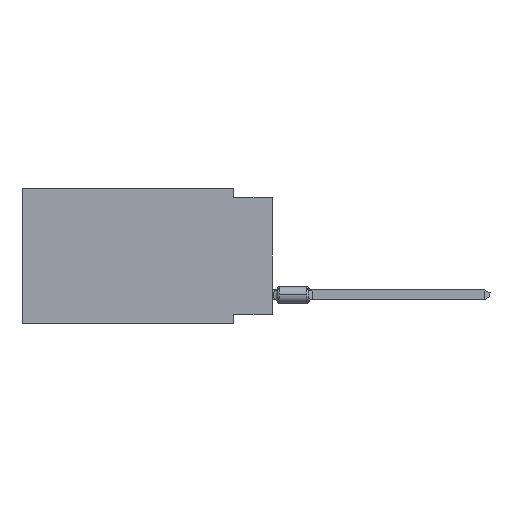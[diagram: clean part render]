
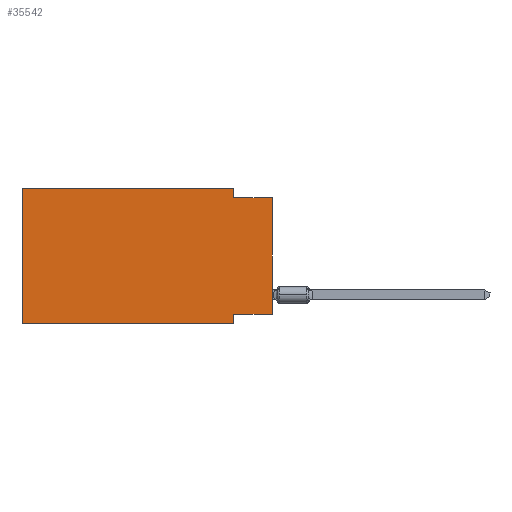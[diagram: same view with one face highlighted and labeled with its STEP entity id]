
A CAD part, left-side view. The second image highlights one B-rep face of the part: STEP entity #35542.
In plain terms, the highlighted planar face has unit normal (-1, 0, 0).
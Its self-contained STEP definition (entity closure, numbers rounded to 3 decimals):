
#1861 = LINE ( 'NONE', #65023, #99935 ) ;
#2441 = CARTESIAN_POINT ( 'NONE',  ( 0., 16.383, 0. ) ) ;
#6344 = VERTEX_POINT ( 'NONE', #110926 ) ;
#9120 = ORIENTED_EDGE ( 'NONE', *, *, #16229, .F. ) ;
#10242 = EDGE_CURVE ( 'NONE', #6344, #46174, #117627, .T. ) ;
#12887 = VERTEX_POINT ( 'NONE', #39884 ) ;
#13921 = VECTOR ( 'NONE', #26841, 1000. ) ;
#15026 = CARTESIAN_POINT ( 'NONE',  ( 0., 2.54, -0.635 ) ) ;
#16229 = EDGE_CURVE ( 'NONE', #12887, #46174, #74353, .T. ) ;
#18744 = DIRECTION ( 'NONE',  ( 0., -1., 0. ) ) ;
#18929 = CARTESIAN_POINT ( 'NONE',  ( 0., 16.383, 0. ) ) ;
#20331 = LINE ( 'NONE', #2441, #113949 ) ;
#21269 = CARTESIAN_POINT ( 'NONE',  ( 0., 2.54, -8.89 ) ) ;
#23142 = VERTEX_POINT ( 'NONE', #36262 ) ;
#25322 = CARTESIAN_POINT ( 'NONE',  ( 0., 16.383, -8.89 ) ) ;
#26738 = DIRECTION ( 'NONE',  ( 0., 0., -1. ) ) ;
#26841 = DIRECTION ( 'NONE',  ( 0., -1., 0. ) ) ;
#28098 = ORIENTED_EDGE ( 'NONE', *, *, #10242, .T. ) ;
#28829 = EDGE_CURVE ( 'NONE', #37947, #23142, #47347, .T. ) ;
#35542 = ADVANCED_FACE ( 'NONE', ( #65366 ), #37944, .F. ) ;
#36262 = CARTESIAN_POINT ( 'NONE',  ( 0., 2.54, 0. ) ) ;
#36494 = CARTESIAN_POINT ( 'NONE',  ( 0., 0., -8.255 ) ) ;
#37944 = PLANE ( 'NONE',  #77385 ) ;
#37947 = VERTEX_POINT ( 'NONE', #81401 ) ;
#39884 = CARTESIAN_POINT ( 'NONE',  ( 0., 2.54, -8.255 ) ) ;
#44779 = DIRECTION ( 'NONE',  ( 0., 0., 1. ) ) ;
#46016 = LINE ( 'NONE', #111509, #105398 ) ;
#46174 = VERTEX_POINT ( 'NONE', #21269 ) ;
#47347 = LINE ( 'NONE', #110507, #92860 ) ;
#48154 = EDGE_CURVE ( 'NONE', #88630, #12887, #46016, .T. ) ;
#50088 = ORIENTED_EDGE ( 'NONE', *, *, #69063, .F. ) ;
#51599 = EDGE_CURVE ( 'NONE', #6344, #37947, #20331, .T. ) ;
#52664 = VECTOR ( 'NONE', #108865, 1000. ) ;
#55258 = DIRECTION ( 'NONE',  ( 0., 0., -1. ) ) ;
#55321 = CARTESIAN_POINT ( 'NONE',  ( 0., 2.54, -8.89 ) ) ;
#55371 = VERTEX_POINT ( 'NONE', #15026 ) ;
#55489 = VERTEX_POINT ( 'NONE', #80514 ) ;
#57009 = ORIENTED_EDGE ( 'NONE', *, *, #108649, .T. ) ;
#62762 = EDGE_CURVE ( 'NONE', #23142, #55371, #72529, .T. ) ;
#65023 = CARTESIAN_POINT ( 'NONE',  ( 0., 0., 0. ) ) ;
#65366 = FACE_OUTER_BOUND ( 'NONE', #105945, .T. ) ;
#69063 = EDGE_CURVE ( 'NONE', #55371, #55489, #88828, .T. ) ;
#71736 = VECTOR ( 'NONE', #18744, 1000. ) ;
#72529 = LINE ( 'NONE', #91586, #52664 ) ;
#74353 = LINE ( 'NONE', #55321, #103791 ) ;
#76889 = ORIENTED_EDGE ( 'NONE', *, *, #62762, .F. ) ;
#77385 = AXIS2_PLACEMENT_3D ( 'NONE', #18929, #82083, #55258 ) ;
#79814 = ORIENTED_EDGE ( 'NONE', *, *, #28829, .F. ) ;
#80514 = CARTESIAN_POINT ( 'NONE',  ( 0., 0., -0.635 ) ) ;
#81401 = CARTESIAN_POINT ( 'NONE',  ( 0., 16.383, 0. ) ) ;
#82083 = DIRECTION ( 'NONE',  ( 1., 0., 0. ) ) ;
#83408 = ORIENTED_EDGE ( 'NONE', *, *, #51599, .F. ) ;
#88630 = VERTEX_POINT ( 'NONE', #36494 ) ;
#88828 = LINE ( 'NONE', #116217, #13921 ) ;
#91586 = CARTESIAN_POINT ( 'NONE',  ( 0., 2.54, 0. ) ) ;
#92860 = VECTOR ( 'NONE', #108753, 1000. ) ;
#92919 = ORIENTED_EDGE ( 'NONE', *, *, #48154, .F. ) ;
#99935 = VECTOR ( 'NONE', #44779, 1000. ) ;
#103702 = DIRECTION ( 'NONE',  ( 0., 0., 1. ) ) ;
#103791 = VECTOR ( 'NONE', #26738, 1000. ) ;
#105398 = VECTOR ( 'NONE', #110351, 1000. ) ;
#105945 = EDGE_LOOP ( 'NONE', ( #57009, #50088, #76889, #79814, #83408, #28098, #9120, #92919 ) ) ;
#108649 = EDGE_CURVE ( 'NONE', #88630, #55489, #1861, .T. ) ;
#108753 = DIRECTION ( 'NONE',  ( 0., -1., 0. ) ) ;
#108865 = DIRECTION ( 'NONE',  ( 0., 0., -1. ) ) ;
#110351 = DIRECTION ( 'NONE',  ( 0., 1., 0. ) ) ;
#110507 = CARTESIAN_POINT ( 'NONE',  ( 0., 16.383, 0. ) ) ;
#110926 = CARTESIAN_POINT ( 'NONE',  ( 0., 16.383, -8.89 ) ) ;
#111509 = CARTESIAN_POINT ( 'NONE',  ( 0., 0., -8.255 ) ) ;
#113949 = VECTOR ( 'NONE', #103702, 1000. ) ;
#116217 = CARTESIAN_POINT ( 'NONE',  ( 0., 0., -0.635 ) ) ;
#117627 = LINE ( 'NONE', #25322, #71736 ) ;
